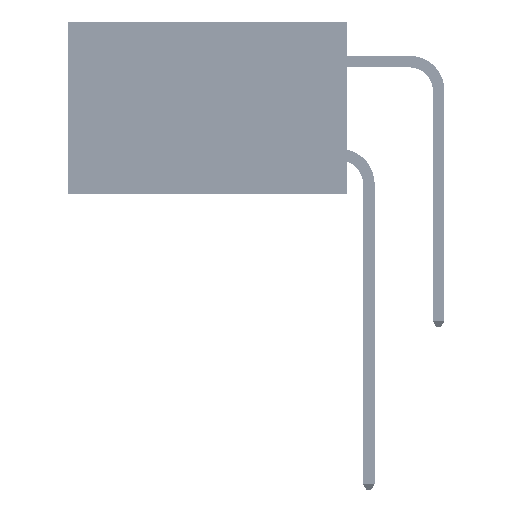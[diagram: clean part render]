
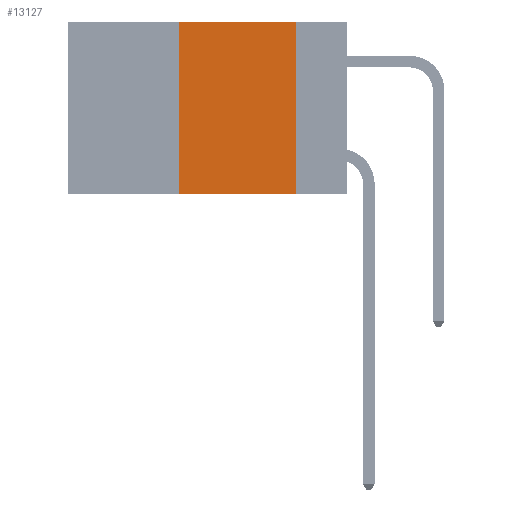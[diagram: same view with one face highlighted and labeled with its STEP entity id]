
A CAD part, left-side view. The second image highlights one B-rep face of the part: STEP entity #13127.
In plain terms, the highlighted planar face has unit normal (-1, 0, 0).
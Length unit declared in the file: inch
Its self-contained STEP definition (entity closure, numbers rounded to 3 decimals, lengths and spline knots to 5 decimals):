
#2482 = FACE_OUTER_BOUND ( 'NONE', #25189, .T. ) ;
#3780 = LINE ( 'NONE', #8760, #31566 ) ;
#5448 = CARTESIAN_POINT ( 'NONE',  ( 0., 0.36, -0.37 ) ) ;
#5960 = ORIENTED_EDGE ( 'NONE', *, *, #30197, .F. ) ;
#7177 = EDGE_CURVE ( 'NONE', #13375, #34573, #3780, .T. ) ;
#8344 = CARTESIAN_POINT ( 'NONE',  ( 0., 0.6, 0. ) ) ;
#8760 = CARTESIAN_POINT ( 'NONE',  ( 0., 0.11, 0. ) ) ;
#11785 = DIRECTION ( 'NONE',  ( 0., 0., 1. ) ) ;
#12016 = CARTESIAN_POINT ( 'NONE',  ( 0., 0.11, 0. ) ) ;
#13127 = ADVANCED_FACE ( 'NONE', ( #2482 ), #22084, .F. ) ;
#13161 = ORIENTED_EDGE ( 'NONE', *, *, #46280, .T. ) ;
#13375 = VERTEX_POINT ( 'NONE', #12016 ) ;
#15338 = AXIS2_PLACEMENT_3D ( 'NONE', #22431, #34786, #26321 ) ;
#16523 = DIRECTION ( 'NONE',  ( 0., 0., -1. ) ) ;
#22084 = PLANE ( 'NONE',  #15338 ) ;
#22431 = CARTESIAN_POINT ( 'NONE',  ( 0., 0.6, 0. ) ) ;
#25189 = EDGE_LOOP ( 'NONE', ( #40270, #48878, #5960, #13161 ) ) ;
#25527 = CARTESIAN_POINT ( 'NONE',  ( 0., 0.6, -0.37 ) ) ;
#26321 = DIRECTION ( 'NONE',  ( 0., 0., -1. ) ) ;
#26416 = LINE ( 'NONE', #51569, #35904 ) ;
#30197 = EDGE_CURVE ( 'NONE', #43146, #44595, #26416, .T. ) ;
#31303 = DIRECTION ( 'NONE',  ( 0., -1., 0. ) ) ;
#31566 = VECTOR ( 'NONE', #16523, 39.37008 ) ;
#32285 = EDGE_CURVE ( 'NONE', #44595, #13375, #45789, .T. ) ;
#33022 = CARTESIAN_POINT ( 'NONE',  ( 0., 0.11, -0.37 ) ) ;
#34565 = CARTESIAN_POINT ( 'NONE',  ( 0., 0.36, 0. ) ) ;
#34573 = VERTEX_POINT ( 'NONE', #33022 ) ;
#34786 = DIRECTION ( 'NONE',  ( 1., 0., 0. ) ) ;
#35873 = VECTOR ( 'NONE', #46168, 39.37008 ) ;
#35904 = VECTOR ( 'NONE', #11785, 39.37008 ) ;
#39018 = LINE ( 'NONE', #25527, #35873 ) ;
#40270 = ORIENTED_EDGE ( 'NONE', *, *, #7177, .F. ) ;
#41955 = VECTOR ( 'NONE', #31303, 39.37008 ) ;
#43146 = VERTEX_POINT ( 'NONE', #5448 ) ;
#44595 = VERTEX_POINT ( 'NONE', #34565 ) ;
#45789 = LINE ( 'NONE', #8344, #41955 ) ;
#46168 = DIRECTION ( 'NONE',  ( 0., -1., 0. ) ) ;
#46280 = EDGE_CURVE ( 'NONE', #43146, #34573, #39018, .T. ) ;
#48878 = ORIENTED_EDGE ( 'NONE', *, *, #32285, .F. ) ;
#51569 = CARTESIAN_POINT ( 'NONE',  ( 0., 0.36, 0. ) ) ;
